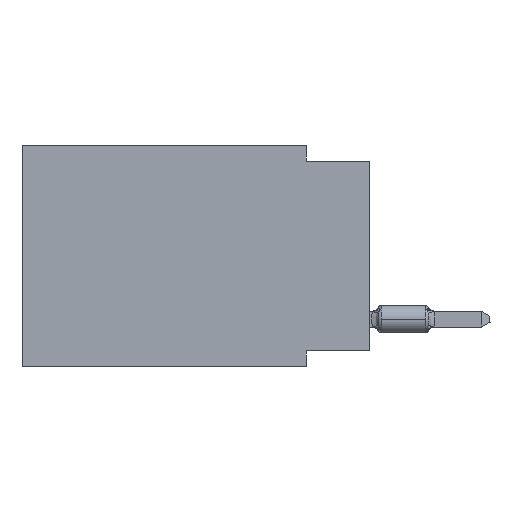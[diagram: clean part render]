
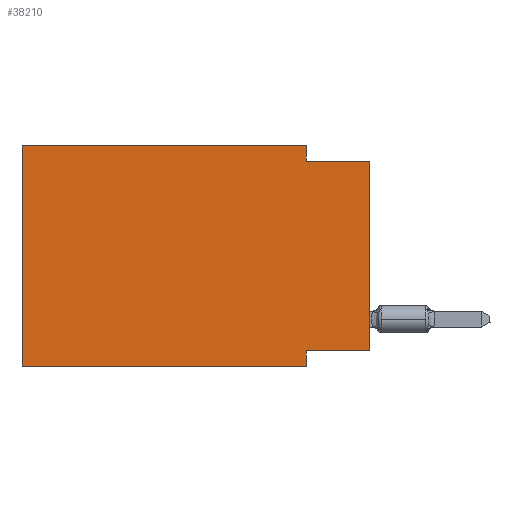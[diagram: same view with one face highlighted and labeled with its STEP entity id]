
A CAD part, left-side view. The second image highlights one B-rep face of the part: STEP entity #38210.
In plain terms, the highlighted planar face has unit normal (-1, 0, 0).
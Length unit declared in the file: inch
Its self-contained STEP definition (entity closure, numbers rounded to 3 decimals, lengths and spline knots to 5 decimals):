
#209 = LINE ( 'NONE', #29178, #22130 ) ;
#289 = VERTEX_POINT ( 'NONE', #14205 ) ;
#409 = DIRECTION ( 'NONE',  ( 0., 0., 1. ) ) ;
#2565 = FACE_OUTER_BOUND ( 'NONE', #33029, .T. ) ;
#2588 = EDGE_CURVE ( 'NONE', #30416, #36723, #3012, .T. ) ;
#3012 = LINE ( 'NONE', #16577, #19303 ) ;
#4611 = EDGE_CURVE ( 'NONE', #27052, #21467, #31027, .T. ) ;
#5130 = DIRECTION ( 'NONE',  ( 1., 0., 0. ) ) ;
#6684 = ORIENTED_EDGE ( 'NONE', *, *, #12456, .F. ) ;
#7317 = ORIENTED_EDGE ( 'NONE', *, *, #17980, .F. ) ;
#7387 = LINE ( 'NONE', #33145, #33380 ) ;
#8006 = ORIENTED_EDGE ( 'NONE', *, *, #2588, .F. ) ;
#8254 = CARTESIAN_POINT ( 'NONE',  ( 0., 0.55, 0. ) ) ;
#8764 = DIRECTION ( 'NONE',  ( 0., 0., 1. ) ) ;
#8909 = ORIENTED_EDGE ( 'NONE', *, *, #4611, .F. ) ;
#11184 = DIRECTION ( 'NONE',  ( 0., 1., 0. ) ) ;
#12063 = LINE ( 'NONE', #24417, #18833 ) ;
#12193 = CARTESIAN_POINT ( 'NONE',  ( 0., 0.1, -0.35 ) ) ;
#12456 = EDGE_CURVE ( 'NONE', #39289, #289, #30559, .T. ) ;
#12490 = ORIENTED_EDGE ( 'NONE', *, *, #28401, .T. ) ;
#14205 = CARTESIAN_POINT ( 'NONE',  ( 0., 0.1, -0.325 ) ) ;
#14288 = CARTESIAN_POINT ( 'NONE',  ( 0., 0.1, -0.025 ) ) ;
#14522 = VECTOR ( 'NONE', #11184, 39.37008 ) ;
#15111 = CARTESIAN_POINT ( 'NONE',  ( 0., 0.55, 0. ) ) ;
#15115 = CARTESIAN_POINT ( 'NONE',  ( 0., 0.1, 0. ) ) ;
#16204 = EDGE_CURVE ( 'NONE', #289, #37837, #209, .T. ) ;
#16577 = CARTESIAN_POINT ( 'NONE',  ( 0., 0.55, 0. ) ) ;
#17273 = LINE ( 'NONE', #37289, #34769 ) ;
#17980 = EDGE_CURVE ( 'NONE', #19306, #27052, #12063, .T. ) ;
#18833 = VECTOR ( 'NONE', #38228, 39.37008 ) ;
#19070 = DIRECTION ( 'NONE',  ( 0., -1., 0. ) ) ;
#19303 = VECTOR ( 'NONE', #409, 39.37008 ) ;
#19306 = VERTEX_POINT ( 'NONE', #15115 ) ;
#19387 = VECTOR ( 'NONE', #19070, 39.37008 ) ;
#19533 = CARTESIAN_POINT ( 'NONE',  ( 0., 0., -0.325 ) ) ;
#20804 = CARTESIAN_POINT ( 'NONE',  ( 0., 0.55, -0.35 ) ) ;
#21467 = VERTEX_POINT ( 'NONE', #38843 ) ;
#21726 = DIRECTION ( 'NONE',  ( 0., 0., -1. ) ) ;
#21944 = CARTESIAN_POINT ( 'NONE',  ( 0., 0., 0. ) ) ;
#22130 = VECTOR ( 'NONE', #28980, 39.37008 ) ;
#24417 = CARTESIAN_POINT ( 'NONE',  ( 0., 0.1, 0. ) ) ;
#25667 = CARTESIAN_POINT ( 'NONE',  ( 0., 0., -0.025 ) ) ;
#27052 = VERTEX_POINT ( 'NONE', #14288 ) ;
#28401 = EDGE_CURVE ( 'NONE', #39289, #21467, #34709, .T. ) ;
#28658 = ORIENTED_EDGE ( 'NONE', *, *, #32235, .T. ) ;
#28980 = DIRECTION ( 'NONE',  ( 0., 0., -1. ) ) ;
#29084 = EDGE_CURVE ( 'NONE', #36723, #19306, #7387, .T. ) ;
#29178 = CARTESIAN_POINT ( 'NONE',  ( 0., 0.1, -0.35 ) ) ;
#30416 = VERTEX_POINT ( 'NONE', #20804 ) ;
#30559 = LINE ( 'NONE', #31191, #14522 ) ;
#31027 = LINE ( 'NONE', #25667, #19387 ) ;
#31191 = CARTESIAN_POINT ( 'NONE',  ( 0., 0., -0.325 ) ) ;
#31600 = ORIENTED_EDGE ( 'NONE', *, *, #16204, .F. ) ;
#32235 = EDGE_CURVE ( 'NONE', #30416, #37837, #17273, .T. ) ;
#33029 = EDGE_LOOP ( 'NONE', ( #12490, #8909, #7317, #41566, #8006, #28658, #31600, #6684 ) ) ;
#33145 = CARTESIAN_POINT ( 'NONE',  ( 0., 0.55, 0. ) ) ;
#33380 = VECTOR ( 'NONE', #33562, 39.37008 ) ;
#33562 = DIRECTION ( 'NONE',  ( 0., -1., 0. ) ) ;
#33665 = DIRECTION ( 'NONE',  ( 0., -1., 0. ) ) ;
#34287 = PLANE ( 'NONE',  #39080 ) ;
#34709 = LINE ( 'NONE', #21944, #34724 ) ;
#34724 = VECTOR ( 'NONE', #8764, 39.37008 ) ;
#34769 = VECTOR ( 'NONE', #33665, 39.37008 ) ;
#36723 = VERTEX_POINT ( 'NONE', #8254 ) ;
#37289 = CARTESIAN_POINT ( 'NONE',  ( 0., 0.55, -0.35 ) ) ;
#37837 = VERTEX_POINT ( 'NONE', #12193 ) ;
#38210 = ADVANCED_FACE ( 'NONE', ( #2565 ), #34287, .F. ) ;
#38228 = DIRECTION ( 'NONE',  ( 0., 0., -1. ) ) ;
#38843 = CARTESIAN_POINT ( 'NONE',  ( 0., 0., -0.025 ) ) ;
#39080 = AXIS2_PLACEMENT_3D ( 'NONE', #15111, #5130, #21726 ) ;
#39289 = VERTEX_POINT ( 'NONE', #19533 ) ;
#41566 = ORIENTED_EDGE ( 'NONE', *, *, #29084, .F. ) ;
